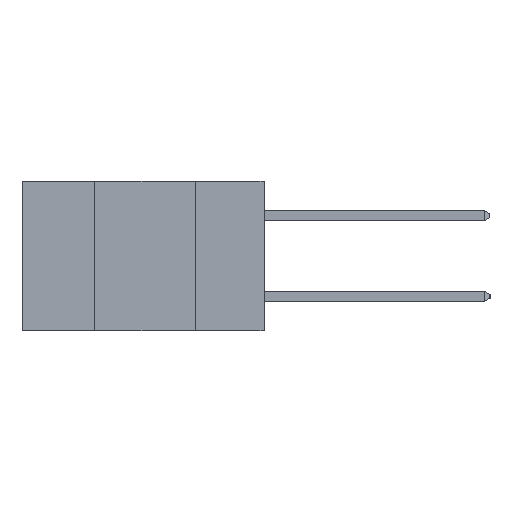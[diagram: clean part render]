
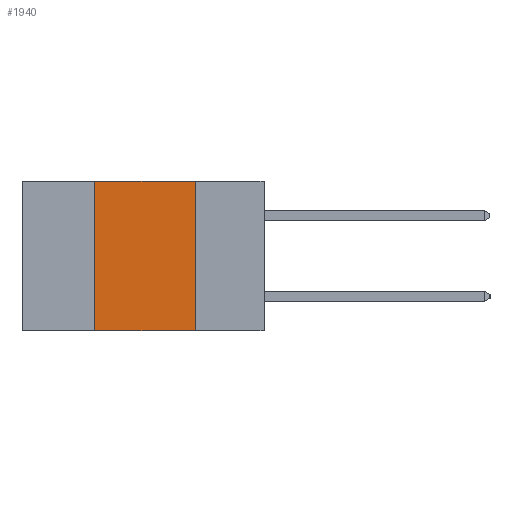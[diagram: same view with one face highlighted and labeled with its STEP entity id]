
A CAD part, left-side view. The second image highlights one B-rep face of the part: STEP entity #1940.
In plain terms, the highlighted planar face has unit normal (-1, 0, 0).
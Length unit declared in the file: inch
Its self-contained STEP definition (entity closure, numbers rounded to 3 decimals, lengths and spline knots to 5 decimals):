
#328 = ORIENTED_EDGE ( 'NONE', *, *, #20631, .F. ) ;
#1007 = DIRECTION ( 'NONE',  ( 0., 0., 1. ) ) ;
#1940 = ADVANCED_FACE ( 'NONE', ( #9163 ), #14058, .F. ) ;
#2518 = LINE ( 'NONE', #12855, #17573 ) ;
#2752 = CARTESIAN_POINT ( 'NONE',  ( 0., 0.6, -0.37 ) ) ;
#4306 = VERTEX_POINT ( 'NONE', #16868 ) ;
#5576 = VECTOR ( 'NONE', #12687, 39.37008 ) ;
#5615 = ORIENTED_EDGE ( 'NONE', *, *, #9616, .T. ) ;
#6038 = VERTEX_POINT ( 'NONE', #6404 ) ;
#6404 = CARTESIAN_POINT ( 'NONE',  ( 0., 0.17, -0.37 ) ) ;
#9163 = FACE_OUTER_BOUND ( 'NONE', #13354, .T. ) ;
#9192 = AXIS2_PLACEMENT_3D ( 'NONE', #14480, #15405, #18371 ) ;
#9252 = VECTOR ( 'NONE', #17199, 39.37008 ) ;
#9370 = CARTESIAN_POINT ( 'NONE',  ( 0., 0.6, 0. ) ) ;
#9616 = EDGE_CURVE ( 'NONE', #9748, #6038, #10871, .T. ) ;
#9674 = ORIENTED_EDGE ( 'NONE', *, *, #22851, .F. ) ;
#9748 = VERTEX_POINT ( 'NONE', #23753 ) ;
#10871 = LINE ( 'NONE', #2752, #5576 ) ;
#12687 = DIRECTION ( 'NONE',  ( 0., -1., 0. ) ) ;
#12855 = CARTESIAN_POINT ( 'NONE',  ( 0., 0.42, -0.37 ) ) ;
#13354 = EDGE_LOOP ( 'NONE', ( #9674, #15514, #328, #5615 ) ) ;
#14058 = PLANE ( 'NONE',  #9192 ) ;
#14083 = CARTESIAN_POINT ( 'NONE',  ( 0., 0.17, 0. ) ) ;
#14480 = CARTESIAN_POINT ( 'NONE',  ( 0., 0.6, 0. ) ) ;
#15405 = DIRECTION ( 'NONE',  ( 1., 0., 0. ) ) ;
#15514 = ORIENTED_EDGE ( 'NONE', *, *, #22526, .F. ) ;
#16868 = CARTESIAN_POINT ( 'NONE',  ( 0., 0.42, 0. ) ) ;
#17199 = DIRECTION ( 'NONE',  ( 0., -1., 0. ) ) ;
#17573 = VECTOR ( 'NONE', #1007, 39.37008 ) ;
#18120 = DIRECTION ( 'NONE',  ( 0., 0., -1. ) ) ;
#18371 = DIRECTION ( 'NONE',  ( 0., 0., -1. ) ) ;
#18987 = LINE ( 'NONE', #9370, #9252 ) ;
#20631 = EDGE_CURVE ( 'NONE', #9748, #4306, #2518, .T. ) ;
#21287 = VECTOR ( 'NONE', #18120, 39.37008 ) ;
#21880 = LINE ( 'NONE', #23690, #21287 ) ;
#22526 = EDGE_CURVE ( 'NONE', #4306, #24714, #18987, .T. ) ;
#22851 = EDGE_CURVE ( 'NONE', #24714, #6038, #21880, .T. ) ;
#23690 = CARTESIAN_POINT ( 'NONE',  ( 0., 0.17, -0.37 ) ) ;
#23753 = CARTESIAN_POINT ( 'NONE',  ( 0., 0.42, -0.37 ) ) ;
#24714 = VERTEX_POINT ( 'NONE', #14083 ) ;
